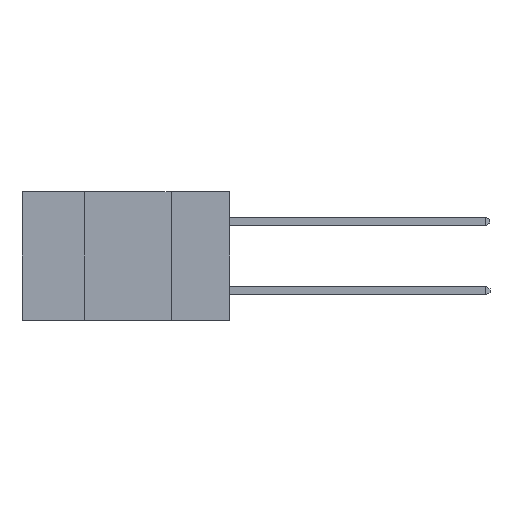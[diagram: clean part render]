
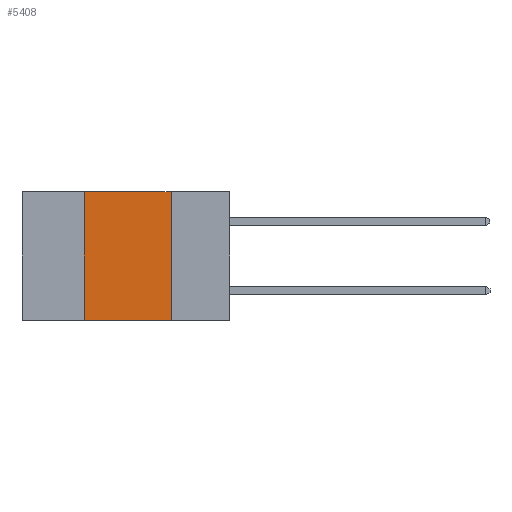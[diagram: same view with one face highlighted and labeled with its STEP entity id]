
A CAD part, left-side view. The second image highlights one B-rep face of the part: STEP entity #5408.
In plain terms, the highlighted planar face has unit normal (-1, 0, 0).
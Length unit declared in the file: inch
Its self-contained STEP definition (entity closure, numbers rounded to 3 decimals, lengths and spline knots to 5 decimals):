
#48 = VECTOR ( 'NONE', #1005, 39.37008 ) ;
#80 = CARTESIAN_POINT ( 'NONE',  ( 0., 0.6, -0.37 ) ) ;
#385 = EDGE_CURVE ( 'NONE', #8471, #4028, #2086, .T. ) ;
#1005 = DIRECTION ( 'NONE',  ( 0., 0., 1. ) ) ;
#1242 = VERTEX_POINT ( 'NONE', #6211 ) ;
#1770 = VECTOR ( 'NONE', #6017, 39.37008 ) ;
#2086 = LINE ( 'NONE', #8488, #7483 ) ;
#2101 = LINE ( 'NONE', #6062, #48 ) ;
#2279 = EDGE_LOOP ( 'NONE', ( #4151, #6341, #7032, #3292 ) ) ;
#2595 = DIRECTION ( 'NONE',  ( 1., 0., 0. ) ) ;
#3292 = ORIENTED_EDGE ( 'NONE', *, *, #6853, .T. ) ;
#3390 = EDGE_CURVE ( 'NONE', #1242, #8471, #4262, .T. ) ;
#3918 = DIRECTION ( 'NONE',  ( 0., 0., -1. ) ) ;
#4023 = VECTOR ( 'NONE', #8024, 39.37008 ) ;
#4028 = VERTEX_POINT ( 'NONE', #5067 ) ;
#4151 = ORIENTED_EDGE ( 'NONE', *, *, #385, .F. ) ;
#4262 = LINE ( 'NONE', #8692, #4023 ) ;
#4362 = CARTESIAN_POINT ( 'NONE',  ( 0., 0.17, 0. ) ) ;
#5067 = CARTESIAN_POINT ( 'NONE',  ( 0., 0.17, -0.37 ) ) ;
#5408 = ADVANCED_FACE ( 'NONE', ( #7528 ), #5562, .F. ) ;
#5562 = PLANE ( 'NONE',  #7013 ) ;
#6017 = DIRECTION ( 'NONE',  ( 0., -1., 0. ) ) ;
#6062 = CARTESIAN_POINT ( 'NONE',  ( 0., 0.42, -0.37 ) ) ;
#6211 = CARTESIAN_POINT ( 'NONE',  ( 0., 0.42, 0. ) ) ;
#6341 = ORIENTED_EDGE ( 'NONE', *, *, #3390, .F. ) ;
#6443 = VERTEX_POINT ( 'NONE', #8388 ) ;
#6839 = CARTESIAN_POINT ( 'NONE',  ( 0., 0.6, 0. ) ) ;
#6853 = EDGE_CURVE ( 'NONE', #6443, #4028, #9165, .T. ) ;
#7013 = AXIS2_PLACEMENT_3D ( 'NONE', #6839, #2595, #7506 ) ;
#7032 = ORIENTED_EDGE ( 'NONE', *, *, #7824, .F. ) ;
#7483 = VECTOR ( 'NONE', #3918, 39.37008 ) ;
#7506 = DIRECTION ( 'NONE',  ( 0., 0., -1. ) ) ;
#7528 = FACE_OUTER_BOUND ( 'NONE', #2279, .T. ) ;
#7824 = EDGE_CURVE ( 'NONE', #6443, #1242, #2101, .T. ) ;
#8024 = DIRECTION ( 'NONE',  ( 0., -1., 0. ) ) ;
#8388 = CARTESIAN_POINT ( 'NONE',  ( 0., 0.42, -0.37 ) ) ;
#8471 = VERTEX_POINT ( 'NONE', #4362 ) ;
#8488 = CARTESIAN_POINT ( 'NONE',  ( 0., 0.17, -0.37 ) ) ;
#8692 = CARTESIAN_POINT ( 'NONE',  ( 0., 0.6, 0. ) ) ;
#9165 = LINE ( 'NONE', #80, #1770 ) ;
